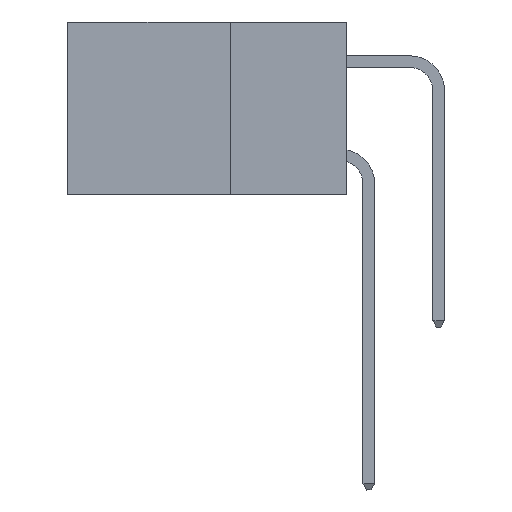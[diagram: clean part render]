
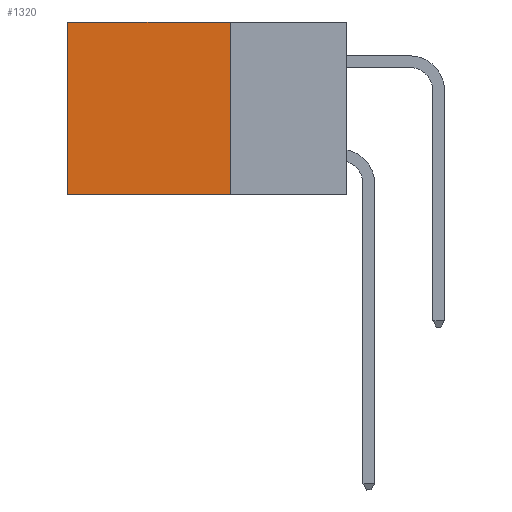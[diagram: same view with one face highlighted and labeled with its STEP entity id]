
A CAD part, left-side view. The second image highlights one B-rep face of the part: STEP entity #1320.
In plain terms, the highlighted planar face has unit normal (-1, 0, 0).
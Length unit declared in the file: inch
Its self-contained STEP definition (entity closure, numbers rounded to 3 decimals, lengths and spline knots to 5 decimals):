
#134 = ORIENTED_EDGE ( 'NONE', *, *, #4129, .T. ) ;
#158 = CARTESIAN_POINT ( 'NONE',  ( 0.2875, 0.25, 0. ) ) ;
#1068 = LINE ( 'NONE', #158, #7341 ) ;
#1320 = ADVANCED_FACE ( 'NONE', ( #4482 ), #5227, .F. ) ;
#1752 = LINE ( 'NONE', #4192, #6432 ) ;
#1907 = EDGE_CURVE ( 'NONE', #14607, #13988, #1752, .T. ) ;
#2679 = CARTESIAN_POINT ( 'NONE',  ( 0.2875, 0.25, -0.37 ) ) ;
#2712 = DIRECTION ( 'NONE',  ( 0., 0., -1. ) ) ;
#3022 = CARTESIAN_POINT ( 'NONE',  ( 0.2875, 0.25, -0.37 ) ) ;
#3414 = EDGE_CURVE ( 'NONE', #13988, #15752, #12884, .T. ) ;
#4062 = DIRECTION ( 'NONE',  ( 0., 1., 0. ) ) ;
#4129 = EDGE_CURVE ( 'NONE', #14607, #4622, #1068, .T. ) ;
#4192 = CARTESIAN_POINT ( 'NONE',  ( 0.2875, 0.25, 0. ) ) ;
#4463 = VECTOR ( 'NONE', #15642, 39.37008 ) ;
#4482 = FACE_OUTER_BOUND ( 'NONE', #14492, .T. ) ;
#4622 = VERTEX_POINT ( 'NONE', #10369 ) ;
#5227 = PLANE ( 'NONE',  #14078 ) ;
#6432 = VECTOR ( 'NONE', #2712, 39.37008 ) ;
#6865 = DIRECTION ( 'NONE',  ( 0., 1., 0. ) ) ;
#7341 = VECTOR ( 'NONE', #4062, 39.37008 ) ;
#7892 = CARTESIAN_POINT ( 'NONE',  ( 0.2875, 0.6, 0. ) ) ;
#7942 = VECTOR ( 'NONE', #6865, 39.37008 ) ;
#8860 = CARTESIAN_POINT ( 'NONE',  ( 0.2875, 0.25, 0. ) ) ;
#9144 = ORIENTED_EDGE ( 'NONE', *, *, #3414, .F. ) ;
#10171 = DIRECTION ( 'NONE',  ( 1., 0., 0. ) ) ;
#10369 = CARTESIAN_POINT ( 'NONE',  ( 0.2875, 0.6, 0. ) ) ;
#10600 = LINE ( 'NONE', #7892, #4463 ) ;
#10892 = DIRECTION ( 'NONE',  ( 0., 0., -1. ) ) ;
#12283 = CARTESIAN_POINT ( 'NONE',  ( 0.2875, 0.6, -0.37 ) ) ;
#12884 = LINE ( 'NONE', #3022, #7942 ) ;
#13389 = ORIENTED_EDGE ( 'NONE', *, *, #1907, .F. ) ;
#13988 = VERTEX_POINT ( 'NONE', #2679 ) ;
#14078 = AXIS2_PLACEMENT_3D ( 'NONE', #14513, #10171, #10892 ) ;
#14492 = EDGE_LOOP ( 'NONE', ( #16240, #9144, #13389, #134 ) ) ;
#14513 = CARTESIAN_POINT ( 'NONE',  ( 0.2875, 0.25, 0. ) ) ;
#14607 = VERTEX_POINT ( 'NONE', #8860 ) ;
#15135 = EDGE_CURVE ( 'NONE', #4622, #15752, #10600, .T. ) ;
#15642 = DIRECTION ( 'NONE',  ( 0., 0., -1. ) ) ;
#15752 = VERTEX_POINT ( 'NONE', #12283 ) ;
#16240 = ORIENTED_EDGE ( 'NONE', *, *, #15135, .T. ) ;
